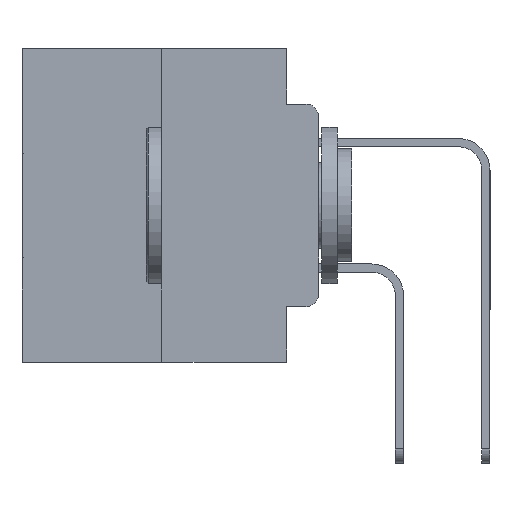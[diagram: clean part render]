
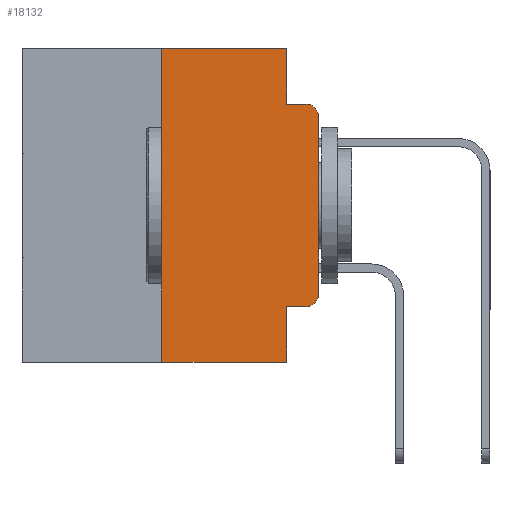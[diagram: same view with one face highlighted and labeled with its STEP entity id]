
A CAD part, left-side view. The second image highlights one B-rep face of the part: STEP entity #18132.
In plain terms, the highlighted planar face has unit normal (-1, 0, 0).
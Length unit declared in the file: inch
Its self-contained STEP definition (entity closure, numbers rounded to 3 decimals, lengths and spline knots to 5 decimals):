
#160 = ORIENTED_EDGE ( 'NONE', *, *, #11277, .F. ) ;
#1020 = LINE ( 'NONE', #15510, #24443 ) ;
#1342 = CIRCLE ( 'NONE', #17669, 0.02 ) ;
#1957 = CARTESIAN_POINT ( 'NONE',  ( 0., 0.051, 0. ) ) ;
#2295 = VECTOR ( 'NONE', #24122, 39.37008 ) ;
#3085 = CARTESIAN_POINT ( 'NONE',  ( 0., 0.473, 0. ) ) ;
#3120 = CARTESIAN_POINT ( 'NONE',  ( 0., 0.473, 0. ) ) ;
#4321 = LINE ( 'NONE', #6954, #10004 ) ;
#4865 = VERTEX_POINT ( 'NONE', #28825 ) ;
#4909 = CIRCLE ( 'NONE', #25446, 0.02 ) ;
#5596 = CARTESIAN_POINT ( 'NONE',  ( 0., 0.051, 0. ) ) ;
#6736 = DIRECTION ( 'NONE',  ( 0., 0., 1. ) ) ;
#6954 = CARTESIAN_POINT ( 'NONE',  ( 0., 0., 0. ) ) ;
#7478 = EDGE_CURVE ( 'NONE', #27972, #19984, #1020, .T. ) ;
#7485 = CARTESIAN_POINT ( 'NONE',  ( 0., 0.051, -0.0885 ) ) ;
#7791 = LINE ( 'NONE', #10829, #19334 ) ;
#8046 = DIRECTION ( 'NONE',  ( 1., 0., 0. ) ) ;
#8558 = CARTESIAN_POINT ( 'NONE',  ( 0., 0.02, -0.3915 ) ) ;
#9139 = EDGE_LOOP ( 'NONE', ( #11122, #14023, #26873, #28344, #160, #25088, #11149, #25918, #22660, #18066 ) ) ;
#9406 = DIRECTION ( 'NONE',  ( -1., 0., 0. ) ) ;
#10004 = VECTOR ( 'NONE', #25505, 39.37008 ) ;
#10829 = CARTESIAN_POINT ( 'NONE',  ( 0., 0.051, -0.4115 ) ) ;
#10924 = DIRECTION ( 'NONE',  ( 0., 0., -1. ) ) ;
#11122 = ORIENTED_EDGE ( 'NONE', *, *, #19034, .T. ) ;
#11149 = ORIENTED_EDGE ( 'NONE', *, *, #25897, .T. ) ;
#11277 = EDGE_CURVE ( 'NONE', #4865, #27972, #27539, .T. ) ;
#11388 = CARTESIAN_POINT ( 'NONE',  ( 0., 0., -0.3915 ) ) ;
#12481 = EDGE_CURVE ( 'NONE', #17618, #14430, #22409, .T. ) ;
#12715 = DIRECTION ( 'NONE',  ( 0., -1., 0. ) ) ;
#13152 = DIRECTION ( 'NONE',  ( 0., -1., 0. ) ) ;
#13384 = EDGE_CURVE ( 'NONE', #23866, #4865, #24866, .T. ) ;
#14023 = ORIENTED_EDGE ( 'NONE', *, *, #22226, .T. ) ;
#14156 = VERTEX_POINT ( 'NONE', #18539 ) ;
#14430 = VERTEX_POINT ( 'NONE', #28631 ) ;
#14467 = VECTOR ( 'NONE', #22955, 39.37008 ) ;
#14758 = VECTOR ( 'NONE', #25920, 39.37008 ) ;
#15510 = CARTESIAN_POINT ( 'NONE',  ( 0., 0.051, 0. ) ) ;
#15836 = EDGE_CURVE ( 'NONE', #26291, #25823, #1342, .T. ) ;
#16913 = FACE_OUTER_BOUND ( 'NONE', #9139, .T. ) ;
#17169 = AXIS2_PLACEMENT_3D ( 'NONE', #3120, #8046, #24115 ) ;
#17618 = VERTEX_POINT ( 'NONE', #24158 ) ;
#17669 = AXIS2_PLACEMENT_3D ( 'NONE', #8558, #24607, #10924 ) ;
#18066 = ORIENTED_EDGE ( 'NONE', *, *, #15836, .T. ) ;
#18132 = ADVANCED_FACE ( 'NONE', ( #16913 ), #26354, .F. ) ;
#18258 = EDGE_CURVE ( 'NONE', #17618, #26291, #7791, .T. ) ;
#18312 = CARTESIAN_POINT ( 'NONE',  ( 0., 0.25, 0. ) ) ;
#18539 = CARTESIAN_POINT ( 'NONE',  ( 0., 0.02, -0.0885 ) ) ;
#18803 = VECTOR ( 'NONE', #6736, 39.37008 ) ;
#19034 = EDGE_CURVE ( 'NONE', #25823, #22017, #4321, .T. ) ;
#19334 = VECTOR ( 'NONE', #13152, 39.37008 ) ;
#19343 = LINE ( 'NONE', #7485, #14758 ) ;
#19984 = VERTEX_POINT ( 'NONE', #22032 ) ;
#21196 = LINE ( 'NONE', #27608, #14467 ) ;
#21386 = VECTOR ( 'NONE', #12715, 39.37008 ) ;
#22017 = VERTEX_POINT ( 'NONE', #29688 ) ;
#22032 = CARTESIAN_POINT ( 'NONE',  ( 0., 0.051, -0.0885 ) ) ;
#22226 = EDGE_CURVE ( 'NONE', #22017, #14156, #4909, .T. ) ;
#22409 = LINE ( 'NONE', #5596, #2295 ) ;
#22660 = ORIENTED_EDGE ( 'NONE', *, *, #18258, .T. ) ;
#22825 = CARTESIAN_POINT ( 'NONE',  ( 0., 0.25, -0.5 ) ) ;
#22955 = DIRECTION ( 'NONE',  ( 0., -1., 0. ) ) ;
#23099 = CARTESIAN_POINT ( 'NONE',  ( 0., 0.02, -0.1085 ) ) ;
#23866 = VERTEX_POINT ( 'NONE', #22825 ) ;
#24115 = DIRECTION ( 'NONE',  ( 0., 0., -1. ) ) ;
#24122 = DIRECTION ( 'NONE',  ( 0., 0., -1. ) ) ;
#24158 = CARTESIAN_POINT ( 'NONE',  ( 0., 0.051, -0.4115 ) ) ;
#24443 = VECTOR ( 'NONE', #24552, 39.37008 ) ;
#24552 = DIRECTION ( 'NONE',  ( 0., 0., -1. ) ) ;
#24607 = DIRECTION ( 'NONE',  ( -1., 0., 0. ) ) ;
#24866 = LINE ( 'NONE', #18312, #18803 ) ;
#25088 = ORIENTED_EDGE ( 'NONE', *, *, #13384, .F. ) ;
#25420 = DIRECTION ( 'NONE',  ( 0., 0., -1. ) ) ;
#25446 = AXIS2_PLACEMENT_3D ( 'NONE', #23099, #9406, #25420 ) ;
#25505 = DIRECTION ( 'NONE',  ( 0., 0., 1. ) ) ;
#25823 = VERTEX_POINT ( 'NONE', #11388 ) ;
#25897 = EDGE_CURVE ( 'NONE', #23866, #14430, #21196, .T. ) ;
#25918 = ORIENTED_EDGE ( 'NONE', *, *, #12481, .F. ) ;
#25920 = DIRECTION ( 'NONE',  ( 0., -1., 0. ) ) ;
#26291 = VERTEX_POINT ( 'NONE', #26957 ) ;
#26354 = PLANE ( 'NONE',  #17169 ) ;
#26873 = ORIENTED_EDGE ( 'NONE', *, *, #29589, .F. ) ;
#26957 = CARTESIAN_POINT ( 'NONE',  ( 0., 0.02, -0.4115 ) ) ;
#27539 = LINE ( 'NONE', #3085, #21386 ) ;
#27608 = CARTESIAN_POINT ( 'NONE',  ( 0., 0.473, -0.5 ) ) ;
#27972 = VERTEX_POINT ( 'NONE', #1957 ) ;
#28344 = ORIENTED_EDGE ( 'NONE', *, *, #7478, .F. ) ;
#28631 = CARTESIAN_POINT ( 'NONE',  ( 0., 0.051, -0.5 ) ) ;
#28825 = CARTESIAN_POINT ( 'NONE',  ( 0., 0.25, 0. ) ) ;
#29589 = EDGE_CURVE ( 'NONE', #19984, #14156, #19343, .T. ) ;
#29688 = CARTESIAN_POINT ( 'NONE',  ( 0., 0., -0.1085 ) ) ;
